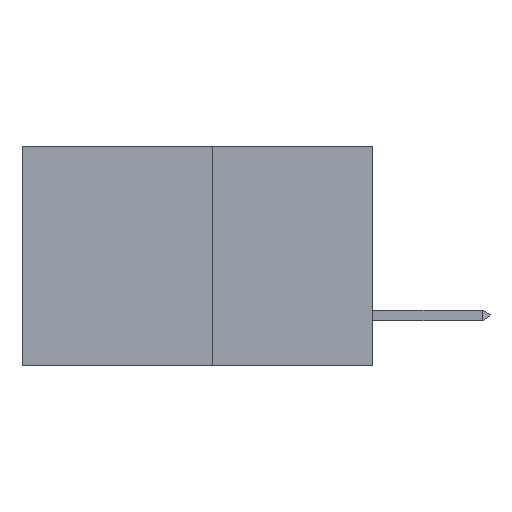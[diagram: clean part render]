
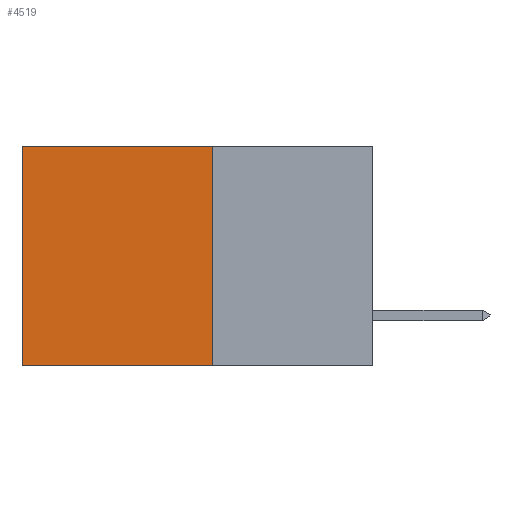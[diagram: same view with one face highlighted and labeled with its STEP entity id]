
A CAD part, left-side view. The second image highlights one B-rep face of the part: STEP entity #4519.
In plain terms, the highlighted planar face has unit normal (-1, 0, 0).
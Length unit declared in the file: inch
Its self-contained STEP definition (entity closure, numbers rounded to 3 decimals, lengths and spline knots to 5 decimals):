
#36 = CARTESIAN_POINT ( 'NONE',  ( 0.277, 0.27, -0.37 ) ) ;
#2398 = ORIENTED_EDGE ( 'NONE', *, *, #8595, .T. ) ;
#3082 = AXIS2_PLACEMENT_3D ( 'NONE', #13522, #12438, #12405 ) ;
#4519 = ADVANCED_FACE ( 'NONE', ( #29212 ), #12569, .F. ) ;
#4568 = DIRECTION ( 'NONE',  ( 0., 1., 0. ) ) ;
#4792 = LINE ( 'NONE', #13964, #16618 ) ;
#6603 = DIRECTION ( 'NONE',  ( 0., 0., -1. ) ) ;
#6953 = CARTESIAN_POINT ( 'NONE',  ( 0.277, 0.27, -0.37 ) ) ;
#7467 = CARTESIAN_POINT ( 'NONE',  ( 0.277, 0.27, 0. ) ) ;
#8595 = EDGE_CURVE ( 'NONE', #24125, #8829, #15384, .T. ) ;
#8829 = VERTEX_POINT ( 'NONE', #17540 ) ;
#8939 = LINE ( 'NONE', #8966, #26823 ) ;
#8966 = CARTESIAN_POINT ( 'NONE',  ( 0.277, 0.59, -0.37 ) ) ;
#9667 = ORIENTED_EDGE ( 'NONE', *, *, #10744, .T. ) ;
#10744 = EDGE_CURVE ( 'NONE', #8829, #11414, #8939, .T. ) ;
#11035 = LINE ( 'NONE', #6953, #22786 ) ;
#11414 = VERTEX_POINT ( 'NONE', #13665 ) ;
#11946 = CARTESIAN_POINT ( 'NONE',  ( 0.277, 0.27, 0. ) ) ;
#12365 = EDGE_LOOP ( 'NONE', ( #9667, #29930, #21237, #2398 ) ) ;
#12405 = DIRECTION ( 'NONE',  ( 0., 0., -1. ) ) ;
#12438 = DIRECTION ( 'NONE',  ( 1., 0., 0. ) ) ;
#12569 = PLANE ( 'NONE',  #3082 ) ;
#13522 = CARTESIAN_POINT ( 'NONE',  ( 0.277, 0.27, -0.37 ) ) ;
#13665 = CARTESIAN_POINT ( 'NONE',  ( 0.277, 0.59, -0.37 ) ) ;
#13964 = CARTESIAN_POINT ( 'NONE',  ( 0.277, 0.27, -0.37 ) ) ;
#15384 = LINE ( 'NONE', #11946, #26950 ) ;
#16357 = DIRECTION ( 'NONE',  ( 0., 0., -1. ) ) ;
#16618 = VECTOR ( 'NONE', #4568, 39.37008 ) ;
#17540 = CARTESIAN_POINT ( 'NONE',  ( 0.277, 0.59, 0. ) ) ;
#21237 = ORIENTED_EDGE ( 'NONE', *, *, #23977, .F. ) ;
#22786 = VECTOR ( 'NONE', #16357, 39.37008 ) ;
#23644 = DIRECTION ( 'NONE',  ( 0., 1., 0. ) ) ;
#23959 = EDGE_CURVE ( 'NONE', #24028, #11414, #4792, .T. ) ;
#23977 = EDGE_CURVE ( 'NONE', #24125, #24028, #11035, .T. ) ;
#24028 = VERTEX_POINT ( 'NONE', #36 ) ;
#24125 = VERTEX_POINT ( 'NONE', #7467 ) ;
#26823 = VECTOR ( 'NONE', #6603, 39.37008 ) ;
#26950 = VECTOR ( 'NONE', #23644, 39.37008 ) ;
#29212 = FACE_OUTER_BOUND ( 'NONE', #12365, .T. ) ;
#29930 = ORIENTED_EDGE ( 'NONE', *, *, #23959, .F. ) ;
